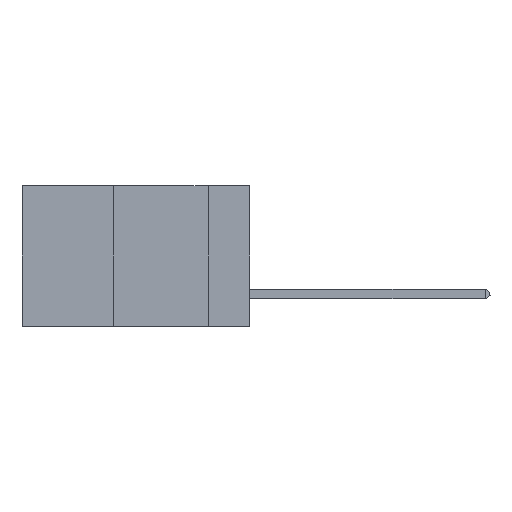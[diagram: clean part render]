
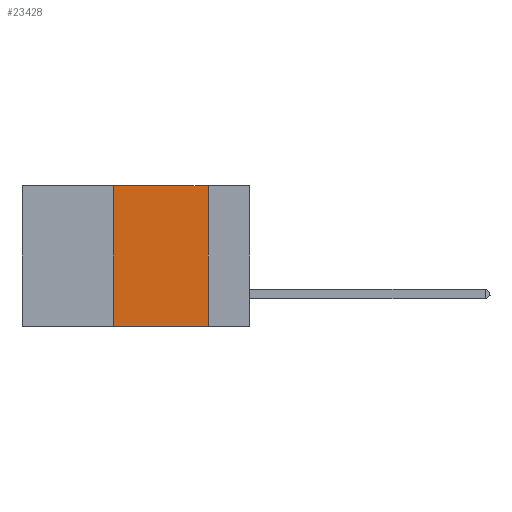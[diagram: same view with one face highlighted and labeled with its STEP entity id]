
A CAD part, left-side view. The second image highlights one B-rep face of the part: STEP entity #23428.
In plain terms, the highlighted planar face has unit normal (-1, 0, 0).
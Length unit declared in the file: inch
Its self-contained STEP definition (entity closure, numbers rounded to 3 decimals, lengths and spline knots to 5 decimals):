
#611 = EDGE_LOOP ( 'NONE', ( #2622, #3636, #7791, #23243 ) ) ;
#2006 = LINE ( 'NONE', #12442, #15524 ) ;
#2516 = LINE ( 'NONE', #19289, #21154 ) ;
#2622 = ORIENTED_EDGE ( 'NONE', *, *, #22192, .F. ) ;
#3183 = DIRECTION ( 'NONE',  ( 0., 0., 1. ) ) ;
#3448 = DIRECTION ( 'NONE',  ( 0., -1., 0. ) ) ;
#3636 = ORIENTED_EDGE ( 'NONE', *, *, #22744, .F. ) ;
#4046 = EDGE_CURVE ( 'NONE', #18960, #18556, #17068, .T. ) ;
#4782 = DIRECTION ( 'NONE',  ( 0., -1., 0. ) ) ;
#6089 = CARTESIAN_POINT ( 'NONE',  ( 0., 0.36, 0. ) ) ;
#6929 = VERTEX_POINT ( 'NONE', #24738 ) ;
#6952 = EDGE_CURVE ( 'NONE', #18960, #6929, #2006, .T. ) ;
#7791 = ORIENTED_EDGE ( 'NONE', *, *, #4046, .F. ) ;
#8660 = VECTOR ( 'NONE', #3183, 39.37008 ) ;
#10728 = CARTESIAN_POINT ( 'NONE',  ( 0., 0.6, 0. ) ) ;
#12442 = CARTESIAN_POINT ( 'NONE',  ( 0., 0.6, -0.37 ) ) ;
#12688 = VECTOR ( 'NONE', #3448, 39.37008 ) ;
#14482 = DIRECTION ( 'NONE',  ( 1., 0., 0. ) ) ;
#14563 = DIRECTION ( 'NONE',  ( 0., 0., -1. ) ) ;
#15524 = VECTOR ( 'NONE', #4782, 39.37008 ) ;
#16627 = CARTESIAN_POINT ( 'NONE',  ( 0., 0.36, 0. ) ) ;
#17068 = LINE ( 'NONE', #16627, #8660 ) ;
#17336 = DIRECTION ( 'NONE',  ( 0., 0., -1. ) ) ;
#17942 = AXIS2_PLACEMENT_3D ( 'NONE', #10728, #14482, #14563 ) ;
#18546 = VERTEX_POINT ( 'NONE', #21304 ) ;
#18556 = VERTEX_POINT ( 'NONE', #6089 ) ;
#18612 = PLANE ( 'NONE',  #17942 ) ;
#18694 = LINE ( 'NONE', #24232, #12688 ) ;
#18960 = VERTEX_POINT ( 'NONE', #24393 ) ;
#19289 = CARTESIAN_POINT ( 'NONE',  ( 0., 0.11, 0. ) ) ;
#21154 = VECTOR ( 'NONE', #17336, 39.37008 ) ;
#21304 = CARTESIAN_POINT ( 'NONE',  ( 0., 0.11, 0. ) ) ;
#22192 = EDGE_CURVE ( 'NONE', #18546, #6929, #2516, .T. ) ;
#22744 = EDGE_CURVE ( 'NONE', #18556, #18546, #18694, .T. ) ;
#23243 = ORIENTED_EDGE ( 'NONE', *, *, #6952, .T. ) ;
#23428 = ADVANCED_FACE ( 'NONE', ( #24704 ), #18612, .F. ) ;
#24232 = CARTESIAN_POINT ( 'NONE',  ( 0., 0.6, 0. ) ) ;
#24393 = CARTESIAN_POINT ( 'NONE',  ( 0., 0.36, -0.37 ) ) ;
#24704 = FACE_OUTER_BOUND ( 'NONE', #611, .T. ) ;
#24738 = CARTESIAN_POINT ( 'NONE',  ( 0., 0.11, -0.37 ) ) ;
